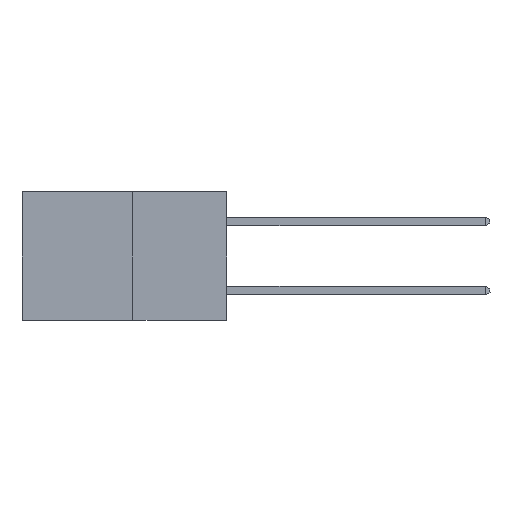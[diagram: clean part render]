
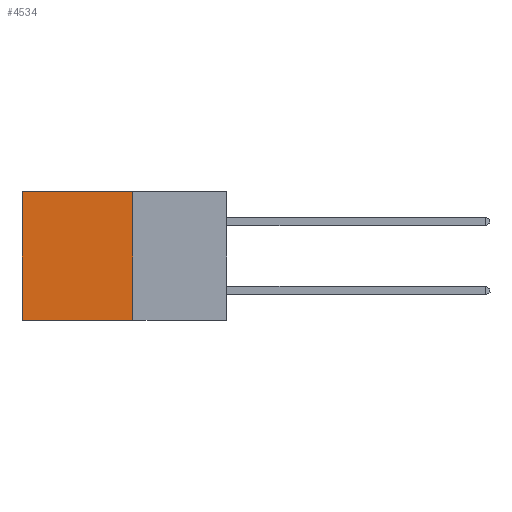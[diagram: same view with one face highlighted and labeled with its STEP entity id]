
A CAD part, left-side view. The second image highlights one B-rep face of the part: STEP entity #4534.
In plain terms, the highlighted planar face has unit normal (-1, 0, 0).
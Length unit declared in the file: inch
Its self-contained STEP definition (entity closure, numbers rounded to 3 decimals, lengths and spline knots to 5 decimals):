
#31 = CARTESIAN_POINT ( 'NONE',  ( 0.277, 0.27, -0.37 ) ) ;
#432 = LINE ( 'NONE', #31, #5862 ) ;
#1772 = CARTESIAN_POINT ( 'NONE',  ( 0.277, 0.59, -0.37 ) ) ;
#1907 = PLANE ( 'NONE',  #23569 ) ;
#2217 = CARTESIAN_POINT ( 'NONE',  ( 0.277, 0.59, -0.37 ) ) ;
#3043 = DIRECTION ( 'NONE',  ( 0., 1., 0. ) ) ;
#3625 = ORIENTED_EDGE ( 'NONE', *, *, #9564, .F. ) ;
#3828 = DIRECTION ( 'NONE',  ( 0., 0., -1. ) ) ;
#3957 = DIRECTION ( 'NONE',  ( 1., 0., 0. ) ) ;
#4333 = VECTOR ( 'NONE', #21463, 39.37008 ) ;
#4534 = ADVANCED_FACE ( 'NONE', ( #23656 ), #1907, .F. ) ;
#5189 = VECTOR ( 'NONE', #3828, 39.37008 ) ;
#5511 = EDGE_CURVE ( 'NONE', #12489, #22811, #23002, .T. ) ;
#5822 = LINE ( 'NONE', #1772, #5189 ) ;
#5862 = VECTOR ( 'NONE', #22108, 39.37008 ) ;
#5983 = VERTEX_POINT ( 'NONE', #24342 ) ;
#9091 = EDGE_LOOP ( 'NONE', ( #11770, #3625, #10298, #16020 ) ) ;
#9392 = CARTESIAN_POINT ( 'NONE',  ( 0.277, 0.27, -0.37 ) ) ;
#9564 = EDGE_CURVE ( 'NONE', #5983, #12978, #15123, .T. ) ;
#10298 = ORIENTED_EDGE ( 'NONE', *, *, #20664, .F. ) ;
#11770 = ORIENTED_EDGE ( 'NONE', *, *, #24606, .T. ) ;
#11824 = VECTOR ( 'NONE', #3043, 39.37008 ) ;
#12489 = VERTEX_POINT ( 'NONE', #14924 ) ;
#12978 = VERTEX_POINT ( 'NONE', #2217 ) ;
#13157 = CARTESIAN_POINT ( 'NONE',  ( 0.277, 0.27, 0. ) ) ;
#14091 = CARTESIAN_POINT ( 'NONE',  ( 0.277, 0.27, -0.37 ) ) ;
#14924 = CARTESIAN_POINT ( 'NONE',  ( 0.277, 0.27, 0. ) ) ;
#15123 = LINE ( 'NONE', #9392, #4333 ) ;
#16020 = ORIENTED_EDGE ( 'NONE', *, *, #5511, .T. ) ;
#18133 = DIRECTION ( 'NONE',  ( 0., 0., -1. ) ) ;
#20664 = EDGE_CURVE ( 'NONE', #12489, #5983, #432, .T. ) ;
#21463 = DIRECTION ( 'NONE',  ( 0., 1., 0. ) ) ;
#22108 = DIRECTION ( 'NONE',  ( 0., 0., -1. ) ) ;
#22681 = CARTESIAN_POINT ( 'NONE',  ( 0.277, 0.59, 0. ) ) ;
#22811 = VERTEX_POINT ( 'NONE', #22681 ) ;
#23002 = LINE ( 'NONE', #13157, #11824 ) ;
#23569 = AXIS2_PLACEMENT_3D ( 'NONE', #14091, #3957, #18133 ) ;
#23656 = FACE_OUTER_BOUND ( 'NONE', #9091, .T. ) ;
#24342 = CARTESIAN_POINT ( 'NONE',  ( 0.277, 0.27, -0.37 ) ) ;
#24606 = EDGE_CURVE ( 'NONE', #22811, #12978, #5822, .T. ) ;
